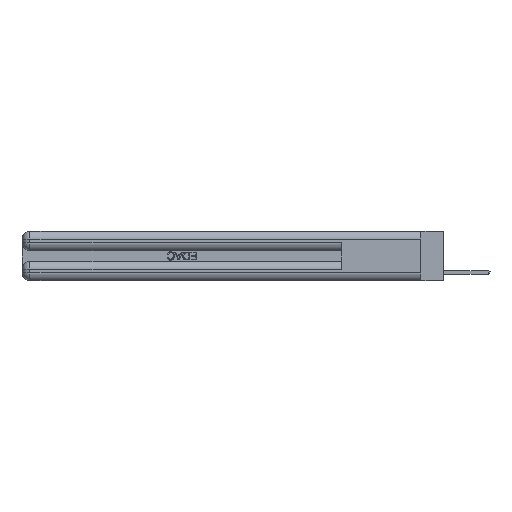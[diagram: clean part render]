
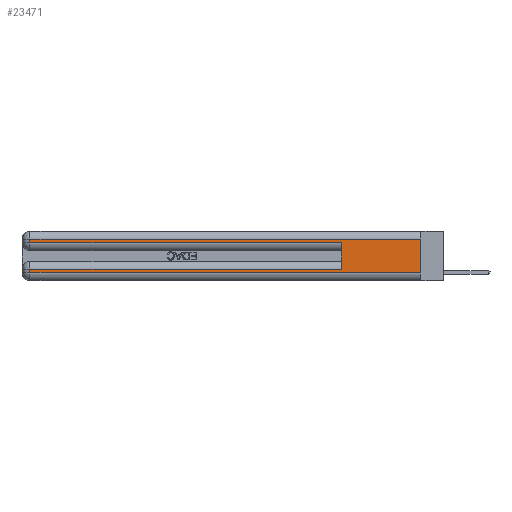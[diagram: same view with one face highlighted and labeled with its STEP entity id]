
A CAD part, left-side view. The second image highlights one B-rep face of the part: STEP entity #23471.
In plain terms, the highlighted planar face has unit normal (-1, 0, 0).
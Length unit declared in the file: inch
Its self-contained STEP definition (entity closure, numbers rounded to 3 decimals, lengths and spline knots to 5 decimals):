
#180 = LINE ( 'NONE', #513, #20460 ) ;
#513 = CARTESIAN_POINT ( 'NONE',  ( 0., 0., 0.31 ) ) ;
#908 = CARTESIAN_POINT ( 'NONE',  ( 0., 0., 0.06 ) ) ;
#1224 = CARTESIAN_POINT ( 'NONE',  ( 0., 2.94, 0.285 ) ) ;
#1505 = CARTESIAN_POINT ( 'NONE',  ( 0., 0., 0.37 ) ) ;
#1596 = PLANE ( 'NONE',  #12345 ) ;
#1851 = VERTEX_POINT ( 'NONE', #16847 ) ;
#2180 = CARTESIAN_POINT ( 'NONE',  ( 0., 2.94, 0.06 ) ) ;
#2408 = ORIENTED_EDGE ( 'NONE', *, *, #12822, .T. ) ;
#2769 = VECTOR ( 'NONE', #26690, 39.37008 ) ;
#3662 = DIRECTION ( 'NONE',  ( 1., 0., 0. ) ) ;
#3755 = ORIENTED_EDGE ( 'NONE', *, *, #9621, .T. ) ;
#4379 = CARTESIAN_POINT ( 'NONE',  ( 0., 0., 0.37 ) ) ;
#4480 = VECTOR ( 'NONE', #22339, 39.37008 ) ;
#4721 = VECTOR ( 'NONE', #24593, 39.37008 ) ;
#5035 = ORIENTED_EDGE ( 'NONE', *, *, #9244, .T. ) ;
#5328 = VERTEX_POINT ( 'NONE', #8013 ) ;
#5375 = LINE ( 'NONE', #11088, #24644 ) ;
#5446 = CARTESIAN_POINT ( 'NONE',  ( 0., 0.6, 0.085 ) ) ;
#6850 = LINE ( 'NONE', #908, #13635 ) ;
#7145 = CARTESIAN_POINT ( 'NONE',  ( 0., 2.94, 0.37 ) ) ;
#8013 = CARTESIAN_POINT ( 'NONE',  ( 0., 2.94, 0.085 ) ) ;
#8036 = DIRECTION ( 'NONE',  ( 0., 0., -1. ) ) ;
#8767 = VECTOR ( 'NONE', #11143, 39.37008 ) ;
#9244 = EDGE_CURVE ( 'NONE', #5328, #21941, #13519, .T. ) ;
#9282 = EDGE_CURVE ( 'NONE', #22094, #5328, #5375, .T. ) ;
#9506 = ORIENTED_EDGE ( 'NONE', *, *, #25477, .T. ) ;
#9621 = EDGE_CURVE ( 'NONE', #23359, #24273, #20237, .T. ) ;
#10477 = VECTOR ( 'NONE', #22107, 39.37008 ) ;
#11088 = CARTESIAN_POINT ( 'NONE',  ( 0., 0., 0.085 ) ) ;
#11143 = DIRECTION ( 'NONE',  ( 0., -1., 0. ) ) ;
#11274 = CARTESIAN_POINT ( 'NONE',  ( 0., 2.94, 0.37 ) ) ;
#11413 = ORIENTED_EDGE ( 'NONE', *, *, #26733, .T. ) ;
#12345 = AXIS2_PLACEMENT_3D ( 'NONE', #1505, #3662, #8036 ) ;
#12822 = EDGE_CURVE ( 'NONE', #21941, #27360, #6850, .T. ) ;
#13519 = LINE ( 'NONE', #11274, #10477 ) ;
#13635 = VECTOR ( 'NONE', #22814, 39.37008 ) ;
#13832 = FACE_OUTER_BOUND ( 'NONE', #16518, .T. ) ;
#15713 = CARTESIAN_POINT ( 'NONE',  ( 0., 2.94, 0.31 ) ) ;
#16202 = LINE ( 'NONE', #17873, #4721 ) ;
#16518 = EDGE_LOOP ( 'NONE', ( #18923, #9506, #11413, #3755, #17267, #27114, #5035, #2408 ) ) ;
#16847 = CARTESIAN_POINT ( 'NONE',  ( 0., 0., 0.31 ) ) ;
#17267 = ORIENTED_EDGE ( 'NONE', *, *, #22672, .F. ) ;
#17873 = CARTESIAN_POINT ( 'NONE',  ( 0., 0.6, 0.145 ) ) ;
#18053 = CARTESIAN_POINT ( 'NONE',  ( 0., 0., 0.06 ) ) ;
#18923 = ORIENTED_EDGE ( 'NONE', *, *, #27289, .F. ) ;
#20237 = LINE ( 'NONE', #25773, #8767 ) ;
#20253 = DIRECTION ( 'NONE',  ( 0., 1., 0. ) ) ;
#20460 = VECTOR ( 'NONE', #20253, 39.37008 ) ;
#20728 = LINE ( 'NONE', #4379, #2769 ) ;
#21378 = LINE ( 'NONE', #7145, #4480 ) ;
#21941 = VERTEX_POINT ( 'NONE', #2180 ) ;
#22094 = VERTEX_POINT ( 'NONE', #5446 ) ;
#22107 = DIRECTION ( 'NONE',  ( 0., 0., -1. ) ) ;
#22339 = DIRECTION ( 'NONE',  ( 0., 0., -1. ) ) ;
#22672 = EDGE_CURVE ( 'NONE', #22094, #24273, #16202, .T. ) ;
#22814 = DIRECTION ( 'NONE',  ( 0., -1., 0. ) ) ;
#23359 = VERTEX_POINT ( 'NONE', #1224 ) ;
#23471 = ADVANCED_FACE ( 'NONE', ( #13832 ), #1596, .F. ) ;
#24273 = VERTEX_POINT ( 'NONE', #25474 ) ;
#24593 = DIRECTION ( 'NONE',  ( 0., 0., 1. ) ) ;
#24644 = VECTOR ( 'NONE', #26383, 39.37008 ) ;
#25474 = CARTESIAN_POINT ( 'NONE',  ( 0., 0.6, 0.285 ) ) ;
#25477 = EDGE_CURVE ( 'NONE', #1851, #27390, #180, .T. ) ;
#25773 = CARTESIAN_POINT ( 'NONE',  ( 0., 0., 0.285 ) ) ;
#26383 = DIRECTION ( 'NONE',  ( 0., 1., 0. ) ) ;
#26690 = DIRECTION ( 'NONE',  ( 0., 0., -1. ) ) ;
#26733 = EDGE_CURVE ( 'NONE', #27390, #23359, #21378, .T. ) ;
#27114 = ORIENTED_EDGE ( 'NONE', *, *, #9282, .T. ) ;
#27289 = EDGE_CURVE ( 'NONE', #1851, #27360, #20728, .T. ) ;
#27360 = VERTEX_POINT ( 'NONE', #18053 ) ;
#27390 = VERTEX_POINT ( 'NONE', #15713 ) ;
